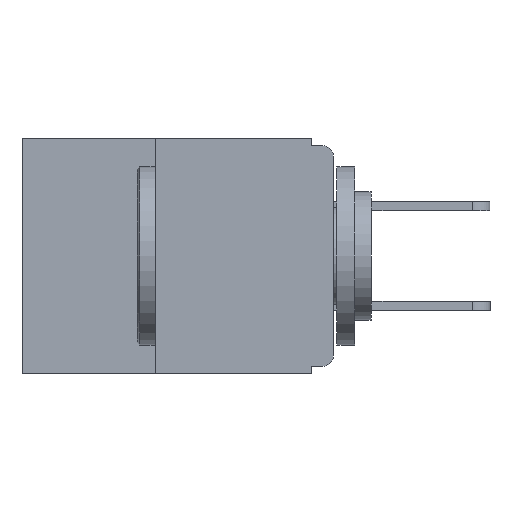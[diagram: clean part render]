
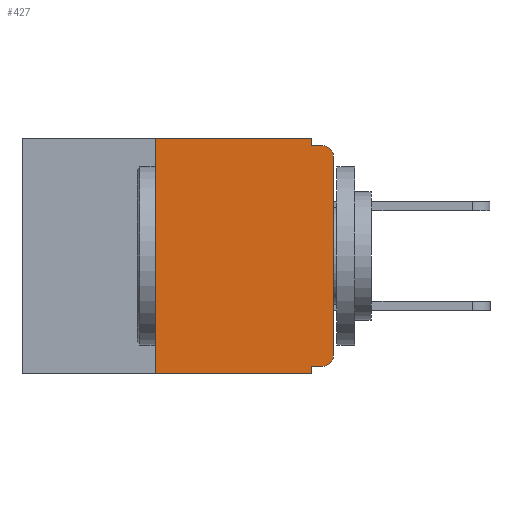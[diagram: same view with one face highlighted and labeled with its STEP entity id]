
A CAD part, left-side view. The second image highlights one B-rep face of the part: STEP entity #427.
In plain terms, the highlighted planar face has unit normal (-1, 0, 0).
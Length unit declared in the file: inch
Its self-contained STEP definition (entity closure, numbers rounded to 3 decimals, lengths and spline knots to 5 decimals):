
#47 = EDGE_CURVE ( 'NONE', #3914, #8042, #3233, .T. ) ;
#427 = ADVANCED_FACE ( 'NONE', ( #11232 ), #7767, .F. ) ;
#486 = DIRECTION ( 'NONE',  ( 0., -1., 0. ) ) ;
#608 = CARTESIAN_POINT ( 'NONE',  ( 0., 0.25, -0.33 ) ) ;
#1187 = ORIENTED_EDGE ( 'NONE', *, *, #11637, .T. ) ;
#1256 = VERTEX_POINT ( 'NONE', #4224 ) ;
#1305 = LINE ( 'NONE', #7160, #8289 ) ;
#1567 = VERTEX_POINT ( 'NONE', #3779 ) ;
#1572 = VECTOR ( 'NONE', #4300, 39.37008 ) ;
#1948 = VERTEX_POINT ( 'NONE', #5303 ) ;
#2069 = CARTESIAN_POINT ( 'NONE',  ( 0., 0.015, -0.01 ) ) ;
#2443 = ORIENTED_EDGE ( 'NONE', *, *, #7245, .F. ) ;
#2500 = CARTESIAN_POINT ( 'NONE',  ( 0., 0.031, 0. ) ) ;
#2614 = EDGE_CURVE ( 'NONE', #1256, #1948, #10899, .T. ) ;
#2665 = VERTEX_POINT ( 'NONE', #2500 ) ;
#2809 = EDGE_LOOP ( 'NONE', ( #1187, #9852, #7897, #5881, #2443, #3583, #10742, #7988, #6458, #9716 ) ) ;
#2928 = VECTOR ( 'NONE', #9453, 39.37008 ) ;
#3063 = CARTESIAN_POINT ( 'NONE',  ( 0., 0.015, -0.305 ) ) ;
#3119 = CARTESIAN_POINT ( 'NONE',  ( 0., 0.031, -0.32 ) ) ;
#3196 = LINE ( 'NONE', #4525, #11053 ) ;
#3233 = LINE ( 'NONE', #4456, #4984 ) ;
#3314 = DIRECTION ( 'NONE',  ( 0., 0., -1. ) ) ;
#3583 = ORIENTED_EDGE ( 'NONE', *, *, #2614, .F. ) ;
#3761 = LINE ( 'NONE', #10147, #5917 ) ;
#3779 = CARTESIAN_POINT ( 'NONE',  ( 0., 0.015, -0.32 ) ) ;
#3900 = DIRECTION ( 'NONE',  ( 0., 0., -1. ) ) ;
#3914 = VERTEX_POINT ( 'NONE', #7496 ) ;
#4008 = CARTESIAN_POINT ( 'NONE',  ( 0., 0.031, -0.33 ) ) ;
#4017 = VERTEX_POINT ( 'NONE', #3119 ) ;
#4224 = CARTESIAN_POINT ( 'NONE',  ( 0., 0.25, -0.33 ) ) ;
#4300 = DIRECTION ( 'NONE',  ( 0., 0., 1. ) ) ;
#4456 = CARTESIAN_POINT ( 'NONE',  ( 0., 0., -0.01 ) ) ;
#4525 = CARTESIAN_POINT ( 'NONE',  ( 0., 0.031, 0. ) ) ;
#4614 = DIRECTION ( 'NONE',  ( 0., 0., 1. ) ) ;
#4930 = EDGE_CURVE ( 'NONE', #1567, #5194, #8649, .T. ) ;
#4958 = CARTESIAN_POINT ( 'NONE',  ( 0., 0.015, -0.025 ) ) ;
#4984 = VECTOR ( 'NONE', #5362, 39.37008 ) ;
#4996 = DIRECTION ( 'NONE',  ( 0., 0., -1. ) ) ;
#5032 = DIRECTION ( 'NONE',  ( 0., 0., -1. ) ) ;
#5194 = VERTEX_POINT ( 'NONE', #11786 ) ;
#5303 = CARTESIAN_POINT ( 'NONE',  ( 0., 0.25, 0. ) ) ;
#5326 = AXIS2_PLACEMENT_3D ( 'NONE', #3063, #9445, #3900 ) ;
#5362 = DIRECTION ( 'NONE',  ( 0., -1., 0. ) ) ;
#5395 = DIRECTION ( 'NONE',  ( 0., 0., -1. ) ) ;
#5630 = VERTEX_POINT ( 'NONE', #11956 ) ;
#5744 = AXIS2_PLACEMENT_3D ( 'NONE', #10580, #9628, #5032 ) ;
#5823 = LINE ( 'NONE', #11722, #10622 ) ;
#5881 = ORIENTED_EDGE ( 'NONE', *, *, #10086, .F. ) ;
#5882 = DIRECTION ( 'NONE',  ( -1., 0., 0. ) ) ;
#5917 = VECTOR ( 'NONE', #4614, 39.37008 ) ;
#6393 = CARTESIAN_POINT ( 'NONE',  ( 0., 0., -0.32 ) ) ;
#6458 = ORIENTED_EDGE ( 'NONE', *, *, #8914, .F. ) ;
#6638 = LINE ( 'NONE', #8315, #8092 ) ;
#7160 = CARTESIAN_POINT ( 'NONE',  ( 0., 0.031, -0.33 ) ) ;
#7245 = EDGE_CURVE ( 'NONE', #1948, #2665, #5823, .T. ) ;
#7453 = AXIS2_PLACEMENT_3D ( 'NONE', #4958, #5882, #4996 ) ;
#7496 = CARTESIAN_POINT ( 'NONE',  ( 0., 0.031, -0.01 ) ) ;
#7767 = PLANE ( 'NONE',  #5744 ) ;
#7897 = ORIENTED_EDGE ( 'NONE', *, *, #47, .F. ) ;
#7988 = ORIENTED_EDGE ( 'NONE', *, *, #9712, .F. ) ;
#8042 = VERTEX_POINT ( 'NONE', #2069 ) ;
#8092 = VECTOR ( 'NONE', #10300, 39.37008 ) ;
#8289 = VECTOR ( 'NONE', #3314, 39.37008 ) ;
#8315 = CARTESIAN_POINT ( 'NONE',  ( 0., 0.437, -0.33 ) ) ;
#8649 = CIRCLE ( 'NONE', #5326, 0.015 ) ;
#8914 = EDGE_CURVE ( 'NONE', #1567, #4017, #10617, .T. ) ;
#9351 = VERTEX_POINT ( 'NONE', #4008 ) ;
#9445 = DIRECTION ( 'NONE',  ( -1., 0., 0. ) ) ;
#9453 = DIRECTION ( 'NONE',  ( 0., 1., 0. ) ) ;
#9628 = DIRECTION ( 'NONE',  ( 1., 0., 0. ) ) ;
#9712 = EDGE_CURVE ( 'NONE', #4017, #9351, #1305, .T. ) ;
#9716 = ORIENTED_EDGE ( 'NONE', *, *, #4930, .T. ) ;
#9852 = ORIENTED_EDGE ( 'NONE', *, *, #11404, .T. ) ;
#10086 = EDGE_CURVE ( 'NONE', #2665, #3914, #3196, .T. ) ;
#10147 = CARTESIAN_POINT ( 'NONE',  ( 0., 0., 0. ) ) ;
#10300 = DIRECTION ( 'NONE',  ( 0., -1., 0. ) ) ;
#10580 = CARTESIAN_POINT ( 'NONE',  ( 0., 0.437, 0. ) ) ;
#10617 = LINE ( 'NONE', #6393, #2928 ) ;
#10622 = VECTOR ( 'NONE', #486, 39.37008 ) ;
#10742 = ORIENTED_EDGE ( 'NONE', *, *, #11641, .T. ) ;
#10899 = LINE ( 'NONE', #608, #1572 ) ;
#11019 = CIRCLE ( 'NONE', #7453, 0.015 ) ;
#11053 = VECTOR ( 'NONE', #5395, 39.37008 ) ;
#11232 = FACE_OUTER_BOUND ( 'NONE', #2809, .T. ) ;
#11404 = EDGE_CURVE ( 'NONE', #5630, #8042, #11019, .T. ) ;
#11637 = EDGE_CURVE ( 'NONE', #5194, #5630, #3761, .T. ) ;
#11641 = EDGE_CURVE ( 'NONE', #1256, #9351, #6638, .T. ) ;
#11722 = CARTESIAN_POINT ( 'NONE',  ( 0., 0.437, 0. ) ) ;
#11786 = CARTESIAN_POINT ( 'NONE',  ( 0., 0., -0.305 ) ) ;
#11956 = CARTESIAN_POINT ( 'NONE',  ( 0., 0., -0.025 ) ) ;
